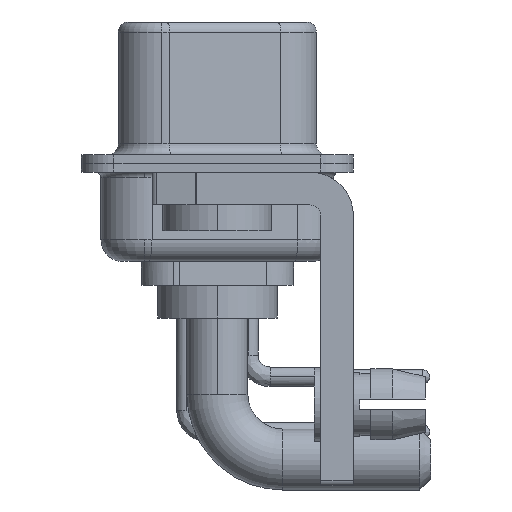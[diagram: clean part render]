
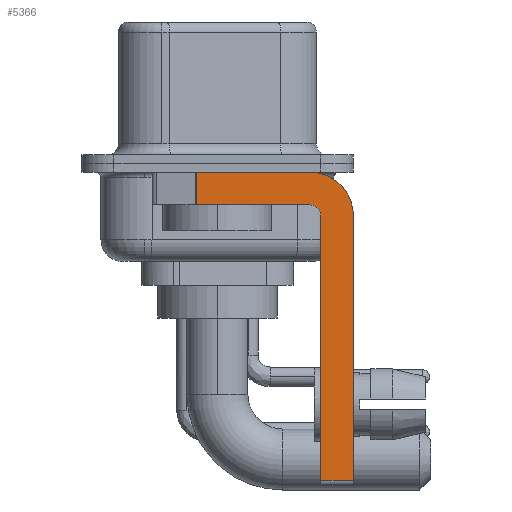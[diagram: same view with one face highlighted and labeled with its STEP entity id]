
A CAD part, left-side view. The second image highlights one B-rep face of the part: STEP entity #5366.
In plain terms, the highlighted planar face has unit normal (-1, 0, 0).
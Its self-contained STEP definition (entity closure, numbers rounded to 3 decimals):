
#49 = VECTOR ( 'NONE', #1695, 1000. ) ;
#192 = EDGE_CURVE ( 'NONE', #1912, #17763, #18798, .T. ) ;
#226 = DIRECTION ( 'NONE',  ( 0., 0., 1. ) ) ;
#261 = CARTESIAN_POINT ( 'NONE',  ( -2.9, -4.25, -0.4 ) ) ;
#365 = DIRECTION ( 'NONE',  ( 0., 1., 0. ) ) ;
#846 = DIRECTION ( 'NONE',  ( 1., 0., 0. ) ) ;
#1501 = CARTESIAN_POINT ( 'NONE',  ( -2.9, -6.25, -2.4 ) ) ;
#1695 = DIRECTION ( 'NONE',  ( 0., 0., -1. ) ) ;
#1815 = CIRCLE ( 'NONE', #13101, 0.5 ) ;
#1912 = VERTEX_POINT ( 'NONE', #22150 ) ;
#2716 = EDGE_CURVE ( 'NONE', #20915, #3351, #5495, .T. ) ;
#2756 = FACE_OUTER_BOUND ( 'NONE', #21414, .T. ) ;
#3028 = DIRECTION ( 'NONE',  ( 1., 0., 0. ) ) ;
#3351 = VERTEX_POINT ( 'NONE', #10253 ) ;
#3382 = ORIENTED_EDGE ( 'NONE', *, *, #3631, .F. ) ;
#3631 = EDGE_CURVE ( 'NONE', #20915, #22756, #13262, .T. ) ;
#3751 = EDGE_CURVE ( 'NONE', #4643, #23522, #1815, .T. ) ;
#4401 = CARTESIAN_POINT ( 'NONE',  ( -2.9, -4.75, -14.55 ) ) ;
#4643 = VERTEX_POINT ( 'NONE', #19717 ) ;
#5366 = ADVANCED_FACE ( 'NONE', ( #2756 ), #10473, .F. ) ;
#5495 = LINE ( 'NONE', #13073, #49 ) ;
#6051 = LINE ( 'NONE', #7946, #11969 ) ;
#7564 = LINE ( 'NONE', #15278, #9916 ) ;
#7708 = EDGE_CURVE ( 'NONE', #13927, #4643, #7564, .T. ) ;
#7946 = CARTESIAN_POINT ( 'NONE',  ( -2.9, -4.25, -14.55 ) ) ;
#9031 = EDGE_CURVE ( 'NONE', #22756, #1912, #22317, .T. ) ;
#9595 = DIRECTION ( 'NONE',  ( 0., -1., 0. ) ) ;
#9916 = VECTOR ( 'NONE', #12994, 1000. ) ;
#10100 = ORIENTED_EDGE ( 'NONE', *, *, #9031, .F. ) ;
#10253 = CARTESIAN_POINT ( 'NONE',  ( -2.9, 0.978, -1.9 ) ) ;
#10473 = PLANE ( 'NONE',  #21218 ) ;
#10753 = DIRECTION ( 'NONE',  ( 0., 0., -1. ) ) ;
#10966 = ORIENTED_EDGE ( 'NONE', *, *, #3751, .F. ) ;
#11433 = AXIS2_PLACEMENT_3D ( 'NONE', #14516, #3028, #10753 ) ;
#11969 = VECTOR ( 'NONE', #9595, 1000. ) ;
#12113 = CARTESIAN_POINT ( 'NONE',  ( -2.9, -4.25, -1.9 ) ) ;
#12994 = DIRECTION ( 'NONE',  ( 0., 0., 1. ) ) ;
#13000 = DIRECTION ( 'NONE',  ( 0., -1., 0. ) ) ;
#13073 = CARTESIAN_POINT ( 'NONE',  ( -2.9, 0.978, -1.9 ) ) ;
#13101 = AXIS2_PLACEMENT_3D ( 'NONE', #23500, #13752, #226 ) ;
#13262 = LINE ( 'NONE', #13381, #21911 ) ;
#13381 = CARTESIAN_POINT ( 'NONE',  ( -2.9, 3., -0.4 ) ) ;
#13617 = EDGE_CURVE ( 'NONE', #23522, #3351, #21735, .T. ) ;
#13752 = DIRECTION ( 'NONE',  ( -1., 0., 0. ) ) ;
#13927 = VERTEX_POINT ( 'NONE', #4401 ) ;
#14243 = ORIENTED_EDGE ( 'NONE', *, *, #7708, .F. ) ;
#14516 = CARTESIAN_POINT ( 'NONE',  ( -2.9, -4.25, -2.4 ) ) ;
#15278 = CARTESIAN_POINT ( 'NONE',  ( -2.9, -4.75, -14.8 ) ) ;
#16592 = VECTOR ( 'NONE', #365, 1000. ) ;
#16944 = CARTESIAN_POINT ( 'NONE',  ( -2.9, -6.25, -14.55 ) ) ;
#17636 = CARTESIAN_POINT ( 'NONE',  ( -2.9, -4.25, -1.9 ) ) ;
#17763 = VERTEX_POINT ( 'NONE', #16944 ) ;
#18148 = CARTESIAN_POINT ( 'NONE',  ( -2.9, -4.25, -2.4 ) ) ;
#18278 = DIRECTION ( 'NONE',  ( 0., 0., -1. ) ) ;
#18798 = LINE ( 'NONE', #1501, #24541 ) ;
#19623 = EDGE_CURVE ( 'NONE', #13927, #17763, #6051, .T. ) ;
#19717 = CARTESIAN_POINT ( 'NONE',  ( -2.9, -4.75, -2.4 ) ) ;
#20915 = VERTEX_POINT ( 'NONE', #24527 ) ;
#21218 = AXIS2_PLACEMENT_3D ( 'NONE', #18148, #846, #18278 ) ;
#21414 = EDGE_LOOP ( 'NONE', ( #3382, #23509, #24966, #10966, #14243, #22288, #23517, #10100 ) ) ;
#21735 = LINE ( 'NONE', #12113, #16592 ) ;
#21911 = VECTOR ( 'NONE', #13000, 1000. ) ;
#22150 = CARTESIAN_POINT ( 'NONE',  ( -2.9, -6.25, -2.4 ) ) ;
#22288 = ORIENTED_EDGE ( 'NONE', *, *, #19623, .T. ) ;
#22317 = CIRCLE ( 'NONE', #11433, 2. ) ;
#22756 = VERTEX_POINT ( 'NONE', #261 ) ;
#23500 = CARTESIAN_POINT ( 'NONE',  ( -2.9, -4.25, -2.4 ) ) ;
#23509 = ORIENTED_EDGE ( 'NONE', *, *, #2716, .T. ) ;
#23517 = ORIENTED_EDGE ( 'NONE', *, *, #192, .F. ) ;
#23522 = VERTEX_POINT ( 'NONE', #17636 ) ;
#24013 = DIRECTION ( 'NONE',  ( 0., 0., -1. ) ) ;
#24527 = CARTESIAN_POINT ( 'NONE',  ( -2.9, 0.978, -0.4 ) ) ;
#24541 = VECTOR ( 'NONE', #24013, 1000. ) ;
#24966 = ORIENTED_EDGE ( 'NONE', *, *, #13617, .F. ) ;
